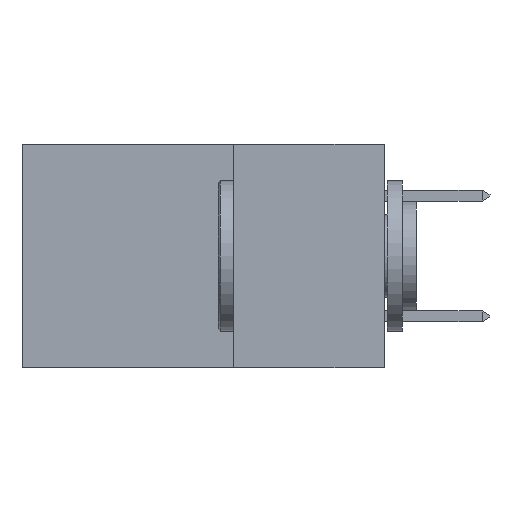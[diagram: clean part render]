
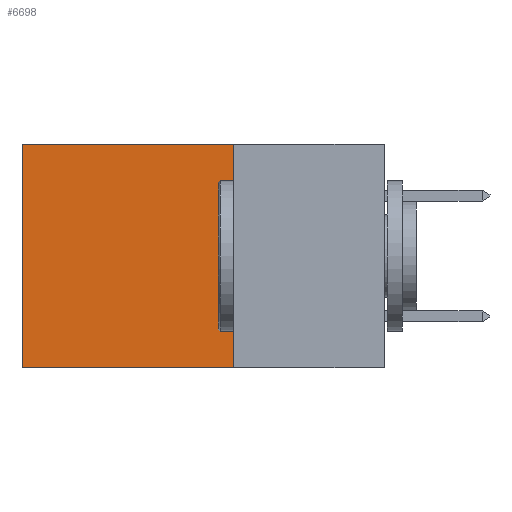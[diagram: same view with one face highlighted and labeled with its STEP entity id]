
A CAD part, left-side view. The second image highlights one B-rep face of the part: STEP entity #6698.
In plain terms, the highlighted planar face has unit normal (-1, 0, 0).
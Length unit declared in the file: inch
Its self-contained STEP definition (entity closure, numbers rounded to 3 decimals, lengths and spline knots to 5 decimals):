
#293 = AXIS2_PLACEMENT_3D ( 'NONE', #8885, #9674, #4973 ) ;
#820 = VECTOR ( 'NONE', #2177, 39.37008 ) ;
#1056 = EDGE_CURVE ( 'NONE', #6114, #2256, #2901, .T. ) ;
#1124 = LINE ( 'NONE', #10351, #820 ) ;
#1292 = EDGE_LOOP ( 'NONE', ( #5255, #5373, #5427, #5434 ) ) ;
#1492 = EDGE_CURVE ( 'NONE', #2776, #2256, #3043, .T. ) ;
#1693 = VERTEX_POINT ( 'NONE', #7074 ) ;
#2177 = DIRECTION ( 'NONE',  ( 0., 1., 0. ) ) ;
#2256 = VERTEX_POINT ( 'NONE', #4276 ) ;
#2466 = DIRECTION ( 'NONE',  ( 0., 0., -1. ) ) ;
#2776 = VERTEX_POINT ( 'NONE', #2970 ) ;
#2901 = LINE ( 'NONE', #10894, #8881 ) ;
#2902 = CARTESIAN_POINT ( 'NONE',  ( 0.2875, 0.6, 0. ) ) ;
#2970 = CARTESIAN_POINT ( 'NONE',  ( 0.2875, 0.6, 0. ) ) ;
#3043 = LINE ( 'NONE', #2902, #8982 ) ;
#4276 = CARTESIAN_POINT ( 'NONE',  ( 0.2875, 0.6, -0.37 ) ) ;
#4973 = DIRECTION ( 'NONE',  ( 0., 0., -1. ) ) ;
#5156 = FACE_OUTER_BOUND ( 'NONE', #1292, .T. ) ;
#5255 = ORIENTED_EDGE ( 'NONE', *, *, #1492, .T. ) ;
#5373 = ORIENTED_EDGE ( 'NONE', *, *, #1056, .F. ) ;
#5427 = ORIENTED_EDGE ( 'NONE', *, *, #9692, .F. ) ;
#5434 = ORIENTED_EDGE ( 'NONE', *, *, #9929, .T. ) ;
#6114 = VERTEX_POINT ( 'NONE', #6951 ) ;
#6698 = ADVANCED_FACE ( 'NONE', ( #5156 ), #7251, .F. ) ;
#6917 = DIRECTION ( 'NONE',  ( 0., 0., -1. ) ) ;
#6951 = CARTESIAN_POINT ( 'NONE',  ( 0.2875, 0.25, -0.37 ) ) ;
#7074 = CARTESIAN_POINT ( 'NONE',  ( 0.2875, 0.25, 0. ) ) ;
#7251 = PLANE ( 'NONE',  #293 ) ;
#7709 = VECTOR ( 'NONE', #6917, 39.37008 ) ;
#8422 = CARTESIAN_POINT ( 'NONE',  ( 0.2875, 0.25, 0. ) ) ;
#8881 = VECTOR ( 'NONE', #8899, 39.37008 ) ;
#8885 = CARTESIAN_POINT ( 'NONE',  ( 0.2875, 0.25, 0. ) ) ;
#8899 = DIRECTION ( 'NONE',  ( 0., 1., 0. ) ) ;
#8982 = VECTOR ( 'NONE', #2466, 39.37008 ) ;
#9674 = DIRECTION ( 'NONE',  ( 1., 0., 0. ) ) ;
#9692 = EDGE_CURVE ( 'NONE', #1693, #6114, #9864, .T. ) ;
#9864 = LINE ( 'NONE', #8422, #7709 ) ;
#9929 = EDGE_CURVE ( 'NONE', #1693, #2776, #1124, .T. ) ;
#10351 = CARTESIAN_POINT ( 'NONE',  ( 0.2875, 0.25, 0. ) ) ;
#10894 = CARTESIAN_POINT ( 'NONE',  ( 0.2875, 0.25, -0.37 ) ) ;
